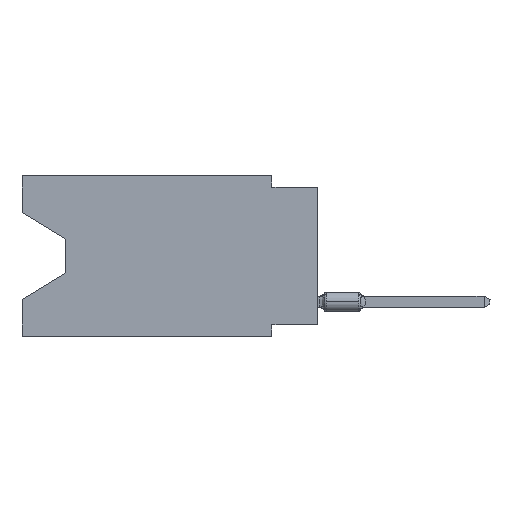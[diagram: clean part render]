
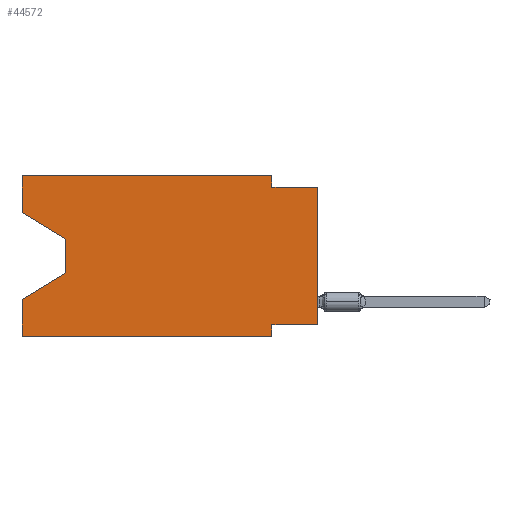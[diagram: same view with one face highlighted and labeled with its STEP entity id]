
A CAD part, left-side view. The second image highlights one B-rep face of the part: STEP entity #44572.
In plain terms, the highlighted planar face has unit normal (-1, 0, 0).
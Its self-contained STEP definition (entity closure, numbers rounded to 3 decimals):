
#262 = DIRECTION ( 'NONE',  ( 0., 0., 1. ) ) ;
#3109 = VERTEX_POINT ( 'NONE', #11169 ) ;
#3560 = VERTEX_POINT ( 'NONE', #60309 ) ;
#3697 = FACE_OUTER_BOUND ( 'NONE', #19384, .T. ) ;
#4432 = EDGE_CURVE ( 'NONE', #31788, #19158, #76603, .T. ) ;
#4595 = VERTEX_POINT ( 'NONE', #35775 ) ;
#4923 = ORIENTED_EDGE ( 'NONE', *, *, #27038, .F. ) ;
#5044 = EDGE_CURVE ( 'NONE', #70058, #63697, #67371, .T. ) ;
#6132 = EDGE_CURVE ( 'NONE', #51186, #80849, #46865, .T. ) ;
#6410 = CARTESIAN_POINT ( 'NONE',  ( 0., 2.54, -8.255 ) ) ;
#6693 = DIRECTION ( 'NONE',  ( 0., -1., 0. ) ) ;
#6838 = CARTESIAN_POINT ( 'NONE',  ( 0., 16.383, -2.038 ) ) ;
#7284 = VERTEX_POINT ( 'NONE', #46975 ) ;
#7665 = CARTESIAN_POINT ( 'NONE',  ( 0., 13.97, -5.385 ) ) ;
#7742 = ORIENTED_EDGE ( 'NONE', *, *, #25188, .F. ) ;
#8379 = AXIS2_PLACEMENT_3D ( 'NONE', #48194, #67931, #22669 ) ;
#8600 = DIRECTION ( 'NONE',  ( 0., 0., -1. ) ) ;
#10176 = ORIENTED_EDGE ( 'NONE', *, *, #64134, .T. ) ;
#10359 = DIRECTION ( 'NONE',  ( 0., 1., 0. ) ) ;
#11169 = CARTESIAN_POINT ( 'NONE',  ( 0., 2.54, 0. ) ) ;
#12043 = ORIENTED_EDGE ( 'NONE', *, *, #45141, .T. ) ;
#12534 = VECTOR ( 'NONE', #50485, 1000. ) ;
#13030 = LINE ( 'NONE', #7665, #66296 ) ;
#15633 = CARTESIAN_POINT ( 'NONE',  ( 0., 0., 0. ) ) ;
#15970 = ORIENTED_EDGE ( 'NONE', *, *, #77262, .F. ) ;
#16476 = VECTOR ( 'NONE', #33562, 1000. ) ;
#16790 = LINE ( 'NONE', #17590, #43954 ) ;
#17590 = CARTESIAN_POINT ( 'NONE',  ( 0., 16.383, 0. ) ) ;
#19158 = VERTEX_POINT ( 'NONE', #55929 ) ;
#19249 = CARTESIAN_POINT ( 'NONE',  ( 0., 16.383, 0. ) ) ;
#19384 = EDGE_LOOP ( 'NONE', ( #58838, #10176, #12043, #4923, #81439, #43871, #15970, #62140, #7742, #55911, #40715, #50779 ) ) ;
#22669 = DIRECTION ( 'NONE',  ( 0., 0., -1. ) ) ;
#23270 = VERTEX_POINT ( 'NONE', #40237 ) ;
#23562 = CARTESIAN_POINT ( 'NONE',  ( 0., 2.54, -0.635 ) ) ;
#25188 = EDGE_CURVE ( 'NONE', #42940, #19158, #56969, .T. ) ;
#27038 = EDGE_CURVE ( 'NONE', #23270, #4595, #56737, .T. ) ;
#28639 = CARTESIAN_POINT ( 'NONE',  ( 0., 13.97, -3.505 ) ) ;
#29126 = DIRECTION ( 'NONE',  ( 0., -0.855, -0.519 ) ) ;
#29922 = CARTESIAN_POINT ( 'NONE',  ( 0., 2.54, -8.89 ) ) ;
#29993 = VECTOR ( 'NONE', #39133, 1000. ) ;
#30327 = LINE ( 'NONE', #36915, #12534 ) ;
#31788 = VERTEX_POINT ( 'NONE', #38072 ) ;
#32251 = CARTESIAN_POINT ( 'NONE',  ( 0., 0., -0.635 ) ) ;
#33562 = DIRECTION ( 'NONE',  ( 0., 0., 1. ) ) ;
#35205 = DIRECTION ( 'NONE',  ( 0., 0., -1. ) ) ;
#35775 = CARTESIAN_POINT ( 'NONE',  ( 0., 16.383, -6.852 ) ) ;
#36103 = VECTOR ( 'NONE', #35205, 1000. ) ;
#36915 = CARTESIAN_POINT ( 'NONE',  ( 0., 16.383, -8.89 ) ) ;
#37106 = VECTOR ( 'NONE', #262, 1000. ) ;
#38072 = CARTESIAN_POINT ( 'NONE',  ( 0., 0., -8.255 ) ) ;
#39133 = DIRECTION ( 'NONE',  ( 0., 0., 1. ) ) ;
#40237 = CARTESIAN_POINT ( 'NONE',  ( 0., 16.383, -8.89 ) ) ;
#40715 = ORIENTED_EDGE ( 'NONE', *, *, #44941, .F. ) ;
#42009 = PLANE ( 'NONE',  #8379 ) ;
#42475 = CARTESIAN_POINT ( 'NONE',  ( 0., 0., -8.255 ) ) ;
#42940 = VERTEX_POINT ( 'NONE', #23562 ) ;
#43871 = ORIENTED_EDGE ( 'NONE', *, *, #5044, .F. ) ;
#43954 = VECTOR ( 'NONE', #60461, 1000. ) ;
#44572 = ADVANCED_FACE ( 'NONE', ( #3697 ), #42009, .F. ) ;
#44941 = EDGE_CURVE ( 'NONE', #3560, #3109, #16790, .T. ) ;
#45141 = EDGE_CURVE ( 'NONE', #7284, #4595, #13030, .T. ) ;
#45571 = DIRECTION ( 'NONE',  ( 0., 0.855, -0.519 ) ) ;
#46865 = LINE ( 'NONE', #79362, #52574 ) ;
#46975 = CARTESIAN_POINT ( 'NONE',  ( 0., 13.97, -5.385 ) ) ;
#48194 = CARTESIAN_POINT ( 'NONE',  ( 0., 16.383, 0. ) ) ;
#48501 = VECTOR ( 'NONE', #55028, 1000. ) ;
#49997 = CARTESIAN_POINT ( 'NONE',  ( 0., 13.97, -3.505 ) ) ;
#50485 = DIRECTION ( 'NONE',  ( 0., -1., 0. ) ) ;
#50779 = ORIENTED_EDGE ( 'NONE', *, *, #62722, .F. ) ;
#51186 = VERTEX_POINT ( 'NONE', #6838 ) ;
#52574 = VECTOR ( 'NONE', #29126, 1000. ) ;
#55028 = DIRECTION ( 'NONE',  ( 0., 0., -1. ) ) ;
#55727 = VECTOR ( 'NONE', #10359, 1000. ) ;
#55911 = ORIENTED_EDGE ( 'NONE', *, *, #56605, .F. ) ;
#55929 = CARTESIAN_POINT ( 'NONE',  ( 0., 0., -0.635 ) ) ;
#56605 = EDGE_CURVE ( 'NONE', #3109, #42940, #62182, .T. ) ;
#56737 = LINE ( 'NONE', #19249, #37106 ) ;
#56969 = LINE ( 'NONE', #32251, #80229 ) ;
#58047 = CARTESIAN_POINT ( 'NONE',  ( 0., 2.54, 0. ) ) ;
#58838 = ORIENTED_EDGE ( 'NONE', *, *, #6132, .T. ) ;
#59928 = LINE ( 'NONE', #28639, #36103 ) ;
#60309 = CARTESIAN_POINT ( 'NONE',  ( 0., 16.383, 0. ) ) ;
#60461 = DIRECTION ( 'NONE',  ( 0., -1., 0. ) ) ;
#62140 = ORIENTED_EDGE ( 'NONE', *, *, #4432, .T. ) ;
#62182 = LINE ( 'NONE', #58047, #80394 ) ;
#62722 = EDGE_CURVE ( 'NONE', #51186, #3560, #76395, .T. ) ;
#63697 = VERTEX_POINT ( 'NONE', #29922 ) ;
#64134 = EDGE_CURVE ( 'NONE', #80849, #7284, #59928, .T. ) ;
#64445 = CARTESIAN_POINT ( 'NONE',  ( 0., 16.383, 0. ) ) ;
#66296 = VECTOR ( 'NONE', #45571, 1000. ) ;
#67371 = LINE ( 'NONE', #78958, #48501 ) ;
#67931 = DIRECTION ( 'NONE',  ( 1., 0., 0. ) ) ;
#70058 = VERTEX_POINT ( 'NONE', #6410 ) ;
#73771 = LINE ( 'NONE', #42475, #55727 ) ;
#76395 = LINE ( 'NONE', #64445, #16476 ) ;
#76603 = LINE ( 'NONE', #15633, #29993 ) ;
#77262 = EDGE_CURVE ( 'NONE', #31788, #70058, #73771, .T. ) ;
#78958 = CARTESIAN_POINT ( 'NONE',  ( 0., 2.54, -8.89 ) ) ;
#79270 = EDGE_CURVE ( 'NONE', #23270, #63697, #30327, .T. ) ;
#79362 = CARTESIAN_POINT ( 'NONE',  ( 0., 16.383, -2.038 ) ) ;
#80229 = VECTOR ( 'NONE', #6693, 1000. ) ;
#80394 = VECTOR ( 'NONE', #8600, 1000. ) ;
#80849 = VERTEX_POINT ( 'NONE', #49997 ) ;
#81439 = ORIENTED_EDGE ( 'NONE', *, *, #79270, .T. ) ;
